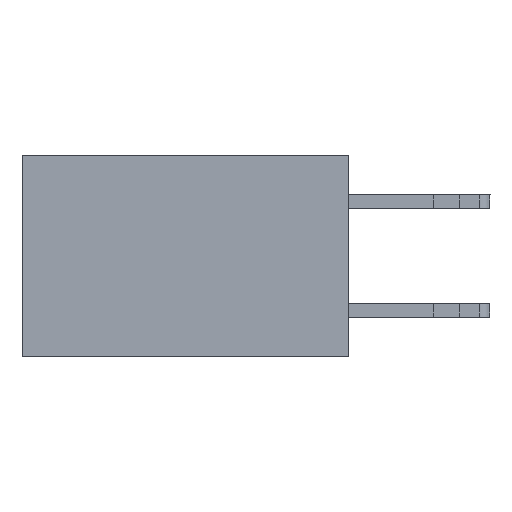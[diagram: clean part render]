
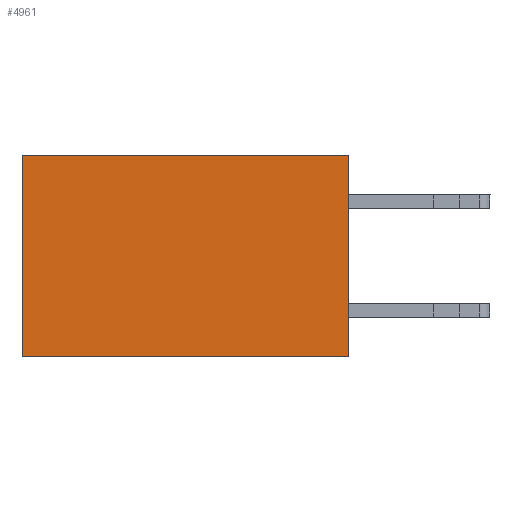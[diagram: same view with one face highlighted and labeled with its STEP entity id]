
A CAD part, left-side view. The second image highlights one B-rep face of the part: STEP entity #4961.
In plain terms, the highlighted planar face has unit normal (-1, 0, 0).
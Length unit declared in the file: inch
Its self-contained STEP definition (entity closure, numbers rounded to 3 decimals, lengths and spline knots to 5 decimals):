
#336 = FACE_OUTER_BOUND ( 'NONE', #5209, .T. ) ;
#918 = ORIENTED_EDGE ( 'NONE', *, *, #3843, .F. ) ;
#1410 = LINE ( 'NONE', #5782, #4053 ) ;
#3470 = DIRECTION ( 'NONE',  ( 0., 0., -1. ) ) ;
#3843 = EDGE_CURVE ( 'NONE', #16450, #18179, #15267, .T. ) ;
#4053 = VECTOR ( 'NONE', #8039, 39.37008 ) ;
#4130 = DIRECTION ( 'NONE',  ( 0., 0., -1. ) ) ;
#4644 = EDGE_CURVE ( 'NONE', #18179, #7369, #1410, .T. ) ;
#4961 = ADVANCED_FACE ( 'NONE', ( #336 ), #11599, .F. ) ;
#4995 = CARTESIAN_POINT ( 'NONE',  ( 0.298, 0., 0. ) ) ;
#5209 = EDGE_LOOP ( 'NONE', ( #20130, #6297, #918, #17438 ) ) ;
#5782 = CARTESIAN_POINT ( 'NONE',  ( 0.298, 0., -0.37 ) ) ;
#6297 = ORIENTED_EDGE ( 'NONE', *, *, #4644, .F. ) ;
#6840 = VECTOR ( 'NONE', #3470, 39.37008 ) ;
#7369 = VERTEX_POINT ( 'NONE', #17828 ) ;
#8039 = DIRECTION ( 'NONE',  ( 0., 1., 0. ) ) ;
#10386 = CARTESIAN_POINT ( 'NONE',  ( 0.298, 0.6, 0. ) ) ;
#11279 = AXIS2_PLACEMENT_3D ( 'NONE', #4995, #14171, #18522 ) ;
#11599 = PLANE ( 'NONE',  #11279 ) ;
#11661 = CARTESIAN_POINT ( 'NONE',  ( 0.298, 0., 0. ) ) ;
#13447 = CARTESIAN_POINT ( 'NONE',  ( 0.298, 0., 0. ) ) ;
#14171 = DIRECTION ( 'NONE',  ( 1., 0., 0. ) ) ;
#15072 = VERTEX_POINT ( 'NONE', #26835 ) ;
#15267 = LINE ( 'NONE', #13447, #21837 ) ;
#15743 = CARTESIAN_POINT ( 'NONE',  ( 0.298, 0., 0. ) ) ;
#16450 = VERTEX_POINT ( 'NONE', #11661 ) ;
#17438 = ORIENTED_EDGE ( 'NONE', *, *, #23614, .T. ) ;
#17828 = CARTESIAN_POINT ( 'NONE',  ( 0.298, 0.6, -0.37 ) ) ;
#18179 = VERTEX_POINT ( 'NONE', #19567 ) ;
#18522 = DIRECTION ( 'NONE',  ( 0., 0., -1. ) ) ;
#19567 = CARTESIAN_POINT ( 'NONE',  ( 0.298, 0., -0.37 ) ) ;
#19805 = EDGE_CURVE ( 'NONE', #15072, #7369, #23611, .T. ) ;
#20130 = ORIENTED_EDGE ( 'NONE', *, *, #19805, .T. ) ;
#21837 = VECTOR ( 'NONE', #4130, 39.37008 ) ;
#22524 = DIRECTION ( 'NONE',  ( 0., 1., 0. ) ) ;
#23611 = LINE ( 'NONE', #10386, #6840 ) ;
#23614 = EDGE_CURVE ( 'NONE', #16450, #15072, #27149, .T. ) ;
#26835 = CARTESIAN_POINT ( 'NONE',  ( 0.298, 0.6, 0. ) ) ;
#27149 = LINE ( 'NONE', #15743, #28212 ) ;
#28212 = VECTOR ( 'NONE', #22524, 39.37008 ) ;
